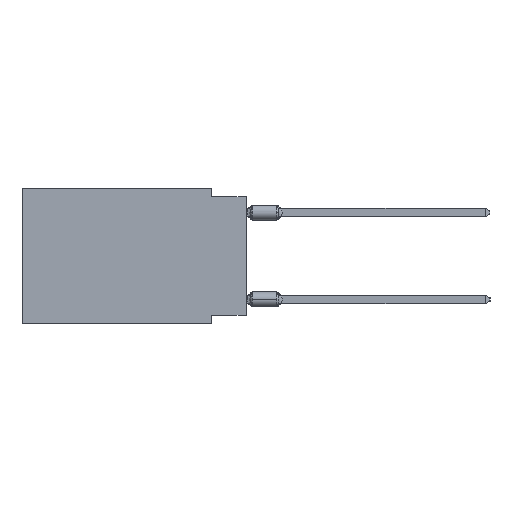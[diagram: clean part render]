
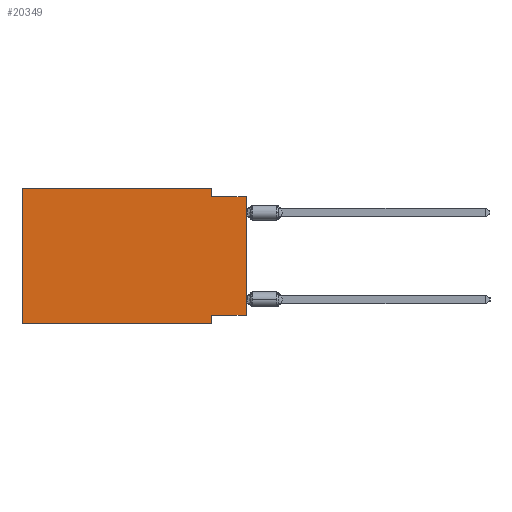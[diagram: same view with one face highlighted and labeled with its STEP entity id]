
A CAD part, left-side view. The second image highlights one B-rep face of the part: STEP entity #20349.
In plain terms, the highlighted planar face has unit normal (-1, 0, 0).
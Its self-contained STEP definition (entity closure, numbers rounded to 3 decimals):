
#1103 = LINE ( 'NONE', #12758, #24599 ) ;
#1937 = VECTOR ( 'NONE', #15542, 1000. ) ;
#2554 = LINE ( 'NONE', #11749, #33119 ) ;
#2784 = EDGE_CURVE ( 'NONE', #30794, #45680, #1103, .T. ) ;
#3775 = CARTESIAN_POINT ( 'NONE',  ( 0., 0., -0.635 ) ) ;
#3847 = VERTEX_POINT ( 'NONE', #19842 ) ;
#4312 = DIRECTION ( 'NONE',  ( 0., -1., 0. ) ) ;
#4323 = CARTESIAN_POINT ( 'NONE',  ( 0., 2.54, -9.271 ) ) ;
#8934 = EDGE_CURVE ( 'NONE', #45014, #3847, #16508, .T. ) ;
#8948 = ORIENTED_EDGE ( 'NONE', *, *, #33644, .F. ) ;
#9662 = CARTESIAN_POINT ( 'NONE',  ( 0., 2.54, -0.635 ) ) ;
#10050 = CARTESIAN_POINT ( 'NONE',  ( 0., 16.383, 0. ) ) ;
#10864 = VERTEX_POINT ( 'NONE', #31022 ) ;
#10882 = VECTOR ( 'NONE', #25911, 1000. ) ;
#10941 = DIRECTION ( 'NONE',  ( 0., 0., -1. ) ) ;
#10968 = LINE ( 'NONE', #39961, #19767 ) ;
#11749 = CARTESIAN_POINT ( 'NONE',  ( 0., 2.54, 0. ) ) ;
#12758 = CARTESIAN_POINT ( 'NONE',  ( 0., 16.383, 0. ) ) ;
#14258 = CARTESIAN_POINT ( 'NONE',  ( 0., 16.383, 0. ) ) ;
#14789 = ORIENTED_EDGE ( 'NONE', *, *, #43877, .F. ) ;
#15542 = DIRECTION ( 'NONE',  ( 0., 1., 0. ) ) ;
#16508 = LINE ( 'NONE', #3775, #32736 ) ;
#18427 = CARTESIAN_POINT ( 'NONE',  ( 0., 16.383, -9.906 ) ) ;
#18574 = ORIENTED_EDGE ( 'NONE', *, *, #8934, .F. ) ;
#18697 = LINE ( 'NONE', #18427, #38282 ) ;
#19555 = ORIENTED_EDGE ( 'NONE', *, *, #23378, .F. ) ;
#19767 = VECTOR ( 'NONE', #32362, 1000. ) ;
#19842 = CARTESIAN_POINT ( 'NONE',  ( 0., 0., -0.635 ) ) ;
#19923 = EDGE_CURVE ( 'NONE', #43311, #10864, #10968, .T. ) ;
#20349 = ADVANCED_FACE ( 'NONE', ( #21161 ), #50210, .F. ) ;
#20889 = ORIENTED_EDGE ( 'NONE', *, *, #2784, .F. ) ;
#21161 = FACE_OUTER_BOUND ( 'NONE', #38296, .T. ) ;
#22679 = DIRECTION ( 'NONE',  ( 0., 0., 1. ) ) ;
#23378 = EDGE_CURVE ( 'NONE', #32123, #45014, #2554, .T. ) ;
#24412 = VERTEX_POINT ( 'NONE', #50644 ) ;
#24599 = VECTOR ( 'NONE', #22679, 1000. ) ;
#25188 = CARTESIAN_POINT ( 'NONE',  ( 0., 0., -9.271 ) ) ;
#25911 = DIRECTION ( 'NONE',  ( 0., 0., 1. ) ) ;
#27131 = VECTOR ( 'NONE', #30246, 1000. ) ;
#30246 = DIRECTION ( 'NONE',  ( 0., -1., 0. ) ) ;
#30794 = VERTEX_POINT ( 'NONE', #32864 ) ;
#31022 = CARTESIAN_POINT ( 'NONE',  ( 0., 2.54, -9.906 ) ) ;
#32123 = VERTEX_POINT ( 'NONE', #40479 ) ;
#32362 = DIRECTION ( 'NONE',  ( 0., 0., -1. ) ) ;
#32736 = VECTOR ( 'NONE', #4312, 1000. ) ;
#32864 = CARTESIAN_POINT ( 'NONE',  ( 0., 16.383, -9.906 ) ) ;
#33119 = VECTOR ( 'NONE', #10941, 1000. ) ;
#33630 = ORIENTED_EDGE ( 'NONE', *, *, #46540, .T. ) ;
#33644 = EDGE_CURVE ( 'NONE', #24412, #43311, #35854, .T. ) ;
#33934 = EDGE_CURVE ( 'NONE', #30794, #10864, #18697, .T. ) ;
#34962 = DIRECTION ( 'NONE',  ( 0., -1., 0. ) ) ;
#35854 = LINE ( 'NONE', #25188, #1937 ) ;
#37980 = DIRECTION ( 'NONE',  ( 0., 0., -1. ) ) ;
#38282 = VECTOR ( 'NONE', #34962, 1000. ) ;
#38296 = EDGE_LOOP ( 'NONE', ( #33630, #18574, #19555, #14789, #20889, #39774, #52599, #8948 ) ) ;
#39774 = ORIENTED_EDGE ( 'NONE', *, *, #33934, .T. ) ;
#39961 = CARTESIAN_POINT ( 'NONE',  ( 0., 2.54, -9.906 ) ) ;
#40479 = CARTESIAN_POINT ( 'NONE',  ( 0., 2.54, 0. ) ) ;
#42451 = LINE ( 'NONE', #46537, #10882 ) ;
#43311 = VERTEX_POINT ( 'NONE', #4323 ) ;
#43877 = EDGE_CURVE ( 'NONE', #45680, #32123, #50889, .T. ) ;
#45014 = VERTEX_POINT ( 'NONE', #9662 ) ;
#45680 = VERTEX_POINT ( 'NONE', #10050 ) ;
#45793 = AXIS2_PLACEMENT_3D ( 'NONE', #45861, #49667, #37980 ) ;
#45861 = CARTESIAN_POINT ( 'NONE',  ( 0., 16.383, 0. ) ) ;
#46537 = CARTESIAN_POINT ( 'NONE',  ( 0., 0., 0. ) ) ;
#46540 = EDGE_CURVE ( 'NONE', #24412, #3847, #42451, .T. ) ;
#49667 = DIRECTION ( 'NONE',  ( 1., 0., 0. ) ) ;
#50210 = PLANE ( 'NONE',  #45793 ) ;
#50644 = CARTESIAN_POINT ( 'NONE',  ( 0., 0., -9.271 ) ) ;
#50889 = LINE ( 'NONE', #14258, #27131 ) ;
#52599 = ORIENTED_EDGE ( 'NONE', *, *, #19923, .F. ) ;
